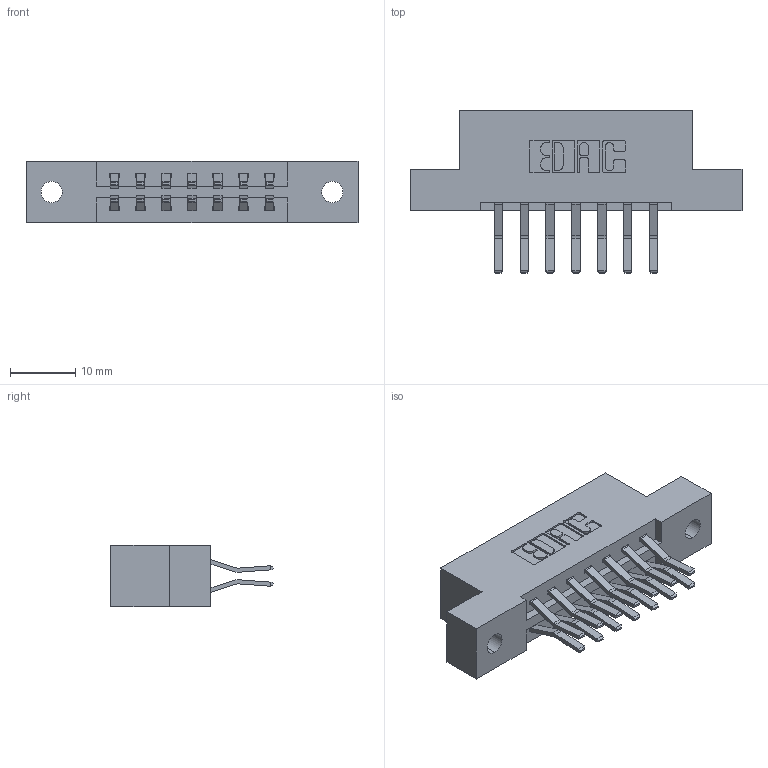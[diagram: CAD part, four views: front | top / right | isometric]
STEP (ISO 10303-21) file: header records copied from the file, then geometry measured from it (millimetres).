
FILE_DESCRIPTION (( 'STEP AP203' ), '1' );
FILE_NAME ('337-014-560-202.STEP', '2019-10-08T12:06:01', ( '' ), ( '' ), 'SwSTEP 2.0', 'SolidWorks 2016', '' );
FILE_SCHEMA (( 'CONFIG_CONTROL_DESIGN' ));
Length unit declared in the file: inch
Products named in the file (3): 337-014-560-202; 345-292-001_560 Tail; 337 Part_Flush Mounting Lugs - 0.128 Dia
Assembly tree (15 placements, depth 2):
  337-014-560-202
    337 Part_Flush Mounting Lugs - 0.128 Dia
    345-292-001_560 Tail  x14
Bounding box: 50.75 x 24.78 x 9.4 mm (x, y, z)
Volume: 4937.6 mm3; surface area: 5234.8 mm2
Topology: 15 solids, 15 shells, 898 faces, 2649 edges, 1746 vertices
Faces by surface type: plane 602, cylinder 296
Entity records: 10045 total; most frequent: CARTESIAN_POINT 1722, ORIENTED_EDGE 1658, DIRECTION 1533, EDGE_CURVE 829, LINE 697, VECTOR 697, VERTEX_POINT 550, AXIS2_PLACEMENT_3D 418
